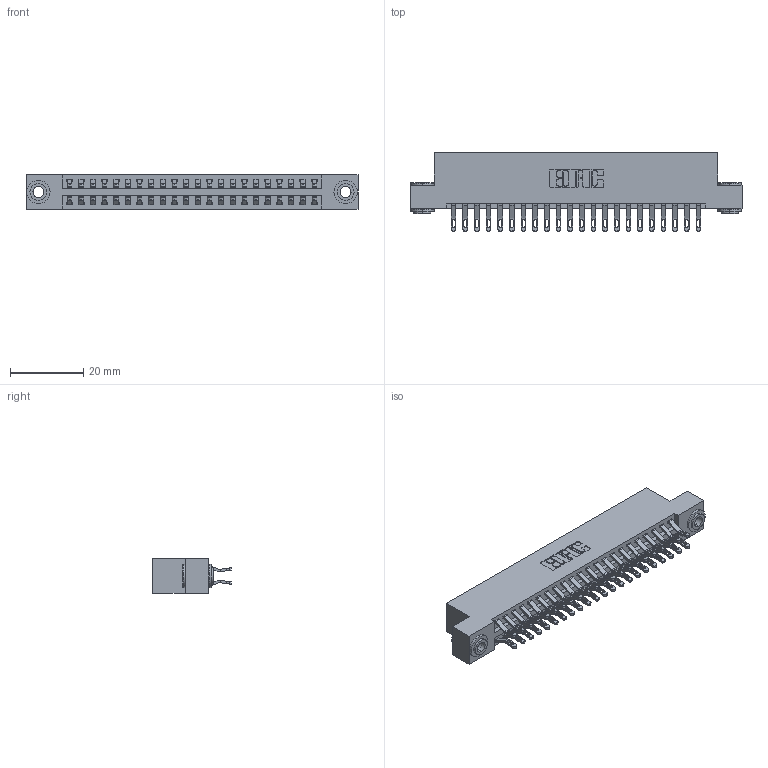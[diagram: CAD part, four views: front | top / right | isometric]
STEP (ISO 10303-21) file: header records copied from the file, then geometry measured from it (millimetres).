
FILE_DESCRIPTION (( 'STEP AP203' ), '1' );
FILE_NAME ('396-044-555-203.STEP', '2018-09-07T04:45:14', ( '' ), ( '' ), 'SwSTEP 2.0', 'SolidWorks 2016', '' );
FILE_SCHEMA (( 'CONFIG_CONTROL_DESIGN' ));
Length unit declared in the file: inch
Products named in the file (4): 345-292-001_555 Tail; 345-250-002_345-250-002-102; 396-044-555-203; 346 Part_Flush Mounting Lugs - 0.156 Dia-TH
Assembly tree (47 placements, depth 2):
  396-044-555-203
    346 Part_Flush Mounting Lugs - 0.156 Dia-TH
    345-292-001_555 Tail  x44
    345-250-002_345-250-002-102  x2
Bounding box: 90.42 x 21.46 x 9.4 mm (x, y, z)
Volume: 8809.1 mm3; surface area: 12463.5 mm2
Topology: 47 solids, 47 shells, 2712 faces, 8457 edges, 5634 vertices
Faces by surface type: plane 1538, cylinder 1166, cone 8
Entity records: 18026 total; most frequent: CARTESIAN_POINT 3009, ORIENTED_EDGE 2906, DIRECTION 2703, EDGE_CURVE 1453, LINE 1189, VECTOR 1189, VERTEX_POINT 966, AXIS2_PLACEMENT_3D 757
